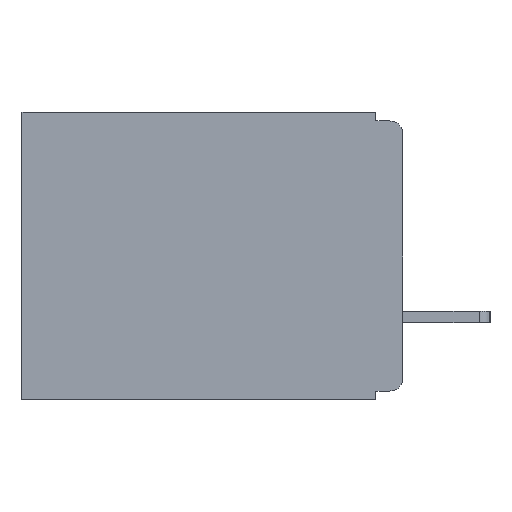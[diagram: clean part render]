
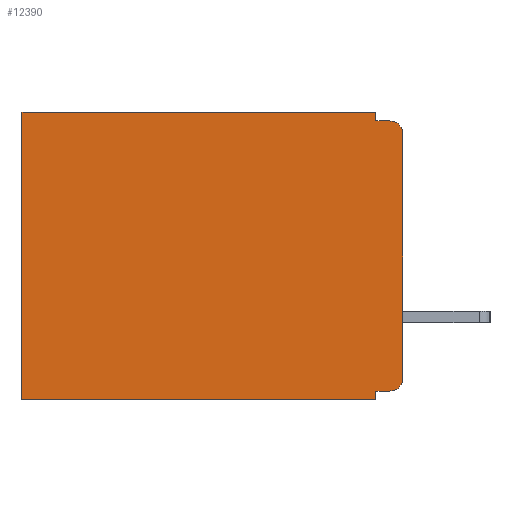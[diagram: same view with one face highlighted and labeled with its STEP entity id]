
A CAD part, left-side view. The second image highlights one B-rep face of the part: STEP entity #12390.
In plain terms, the highlighted planar face has unit normal (-1, 0, 0).
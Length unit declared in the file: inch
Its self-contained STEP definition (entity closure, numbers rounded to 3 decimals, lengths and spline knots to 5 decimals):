
#269 = VECTOR ( 'NONE', #4002, 39.37008 ) ;
#421 = CARTESIAN_POINT ( 'NONE',  ( 0.3, 0.015, -0.32 ) ) ;
#537 = CARTESIAN_POINT ( 'NONE',  ( 0.3, 0.031, -0.01 ) ) ;
#623 = DIRECTION ( 'NONE',  ( 0., 1., 0. ) ) ;
#1016 = VERTEX_POINT ( 'NONE', #2867 ) ;
#1159 = EDGE_CURVE ( 'NONE', #6312, #7584, #10662, .T. ) ;
#1481 = CARTESIAN_POINT ( 'NONE',  ( 0.3, 0., -0.33 ) ) ;
#1645 = EDGE_CURVE ( 'NONE', #7828, #7584, #13724, .T. ) ;
#1833 = EDGE_CURVE ( 'NONE', #1016, #10822, #3444, .T. ) ;
#1849 = VECTOR ( 'NONE', #10338, 39.37008 ) ;
#1900 = VERTEX_POINT ( 'NONE', #421 ) ;
#1949 = EDGE_CURVE ( 'NONE', #6426, #6312, #8142, .T. ) ;
#2030 = CARTESIAN_POINT ( 'NONE',  ( 0.3, 0., -0.025 ) ) ;
#2153 = DIRECTION ( 'NONE',  ( 0., 0., -1. ) ) ;
#2418 = ORIENTED_EDGE ( 'NONE', *, *, #2976, .F. ) ;
#2485 = ORIENTED_EDGE ( 'NONE', *, *, #6458, .T. ) ;
#2760 = FACE_OUTER_BOUND ( 'NONE', #13428, .T. ) ;
#2828 = DIRECTION ( 'NONE',  ( 1., 0., 0. ) ) ;
#2867 = CARTESIAN_POINT ( 'NONE',  ( 0.3, 0.031, 0. ) ) ;
#2869 = ORIENTED_EDGE ( 'NONE', *, *, #1645, .T. ) ;
#2923 = ORIENTED_EDGE ( 'NONE', *, *, #15508, .T. ) ;
#2976 = EDGE_CURVE ( 'NONE', #9250, #5532, #13850, .T. ) ;
#3064 = AXIS2_PLACEMENT_3D ( 'NONE', #11427, #2828, #11474 ) ;
#3134 = CIRCLE ( 'NONE', #11631, 0.015 ) ;
#3245 = AXIS2_PLACEMENT_3D ( 'NONE', #14032, #7699, #13592 ) ;
#3444 = LINE ( 'NONE', #5745, #3858 ) ;
#3838 = EDGE_CURVE ( 'NONE', #10822, #11351, #4952, .T. ) ;
#3858 = VECTOR ( 'NONE', #11877, 39.37008 ) ;
#3916 = CIRCLE ( 'NONE', #3245, 0.015 ) ;
#4002 = DIRECTION ( 'NONE',  ( 0., 1., 0. ) ) ;
#4784 = ORIENTED_EDGE ( 'NONE', *, *, #3838, .F. ) ;
#4952 = LINE ( 'NONE', #5349, #11860 ) ;
#5349 = CARTESIAN_POINT ( 'NONE',  ( 0.3, 0., -0.01 ) ) ;
#5421 = VECTOR ( 'NONE', #623, 39.37008 ) ;
#5532 = VERTEX_POINT ( 'NONE', #15065 ) ;
#5572 = EDGE_CURVE ( 'NONE', #1900, #6426, #9967, .T. ) ;
#5710 = CARTESIAN_POINT ( 'NONE',  ( 0.3, 0., 0. ) ) ;
#5745 = CARTESIAN_POINT ( 'NONE',  ( 0.3, 0.031, 0. ) ) ;
#5785 = EDGE_CURVE ( 'NONE', #9250, #11351, #3134, .T. ) ;
#5820 = CARTESIAN_POINT ( 'NONE',  ( 0.3, 0.437, 0. ) ) ;
#6312 = VERTEX_POINT ( 'NONE', #6860 ) ;
#6426 = VERTEX_POINT ( 'NONE', #10110 ) ;
#6458 = EDGE_CURVE ( 'NONE', #1900, #5532, #3916, .T. ) ;
#6815 = DIRECTION ( 'NONE',  ( 0., 1., 0. ) ) ;
#6860 = CARTESIAN_POINT ( 'NONE',  ( 0.3, 0.031, -0.33 ) ) ;
#7368 = VECTOR ( 'NONE', #13089, 39.37008 ) ;
#7386 = VECTOR ( 'NONE', #6815, 39.37008 ) ;
#7484 = CARTESIAN_POINT ( 'NONE',  ( 0.3, 0., -0.32 ) ) ;
#7584 = VERTEX_POINT ( 'NONE', #9109 ) ;
#7699 = DIRECTION ( 'NONE',  ( -1., 0., 0. ) ) ;
#7828 = VERTEX_POINT ( 'NONE', #5820 ) ;
#7937 = DIRECTION ( 'NONE',  ( 0., -1., 0. ) ) ;
#8142 = LINE ( 'NONE', #8643, #1849 ) ;
#8218 = CARTESIAN_POINT ( 'NONE',  ( 0.3, 0.015, -0.01 ) ) ;
#8643 = CARTESIAN_POINT ( 'NONE',  ( 0.3, 0.031, -0.33 ) ) ;
#9109 = CARTESIAN_POINT ( 'NONE',  ( 0.3, 0.437, -0.33 ) ) ;
#9250 = VERTEX_POINT ( 'NONE', #2030 ) ;
#9967 = LINE ( 'NONE', #7484, #269 ) ;
#10110 = CARTESIAN_POINT ( 'NONE',  ( 0.3, 0.031, -0.32 ) ) ;
#10338 = DIRECTION ( 'NONE',  ( 0., 0., -1. ) ) ;
#10531 = CARTESIAN_POINT ( 'NONE',  ( 0.3, 0., -0.33 ) ) ;
#10662 = LINE ( 'NONE', #10531, #7386 ) ;
#10822 = VERTEX_POINT ( 'NONE', #537 ) ;
#11351 = VERTEX_POINT ( 'NONE', #8218 ) ;
#11383 = DIRECTION ( 'NONE',  ( 0., 0., -1. ) ) ;
#11427 = CARTESIAN_POINT ( 'NONE',  ( 0.3, 0., -0.33 ) ) ;
#11474 = DIRECTION ( 'NONE',  ( 0., 0., -1. ) ) ;
#11631 = AXIS2_PLACEMENT_3D ( 'NONE', #13044, #12209, #11383 ) ;
#11860 = VECTOR ( 'NONE', #7937, 39.37008 ) ;
#11877 = DIRECTION ( 'NONE',  ( 0., 0., -1. ) ) ;
#12209 = DIRECTION ( 'NONE',  ( -1., 0., 0. ) ) ;
#12390 = ADVANCED_FACE ( 'NONE', ( #2760 ), #14868, .F. ) ;
#12622 = ORIENTED_EDGE ( 'NONE', *, *, #1159, .F. ) ;
#12818 = ORIENTED_EDGE ( 'NONE', *, *, #5785, .T. ) ;
#13044 = CARTESIAN_POINT ( 'NONE',  ( 0.3, 0.015, -0.025 ) ) ;
#13089 = DIRECTION ( 'NONE',  ( 0., 0., -1. ) ) ;
#13428 = EDGE_LOOP ( 'NONE', ( #2418, #12818, #4784, #15114, #2923, #2869, #12622, #13589, #14193, #2485 ) ) ;
#13589 = ORIENTED_EDGE ( 'NONE', *, *, #1949, .F. ) ;
#13592 = DIRECTION ( 'NONE',  ( 0., 0., -1. ) ) ;
#13724 = LINE ( 'NONE', #14481, #7368 ) ;
#13850 = LINE ( 'NONE', #1481, #14209 ) ;
#14032 = CARTESIAN_POINT ( 'NONE',  ( 0.3, 0.015, -0.305 ) ) ;
#14193 = ORIENTED_EDGE ( 'NONE', *, *, #5572, .F. ) ;
#14209 = VECTOR ( 'NONE', #2153, 39.37008 ) ;
#14481 = CARTESIAN_POINT ( 'NONE',  ( 0.3, 0.437, -0.33 ) ) ;
#14868 = PLANE ( 'NONE',  #3064 ) ;
#14947 = LINE ( 'NONE', #5710, #5421 ) ;
#15065 = CARTESIAN_POINT ( 'NONE',  ( 0.3, 0., -0.305 ) ) ;
#15114 = ORIENTED_EDGE ( 'NONE', *, *, #1833, .F. ) ;
#15508 = EDGE_CURVE ( 'NONE', #1016, #7828, #14947, .T. ) ;
